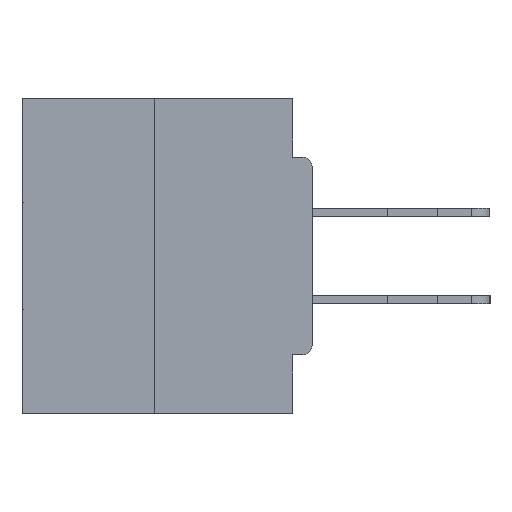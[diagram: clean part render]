
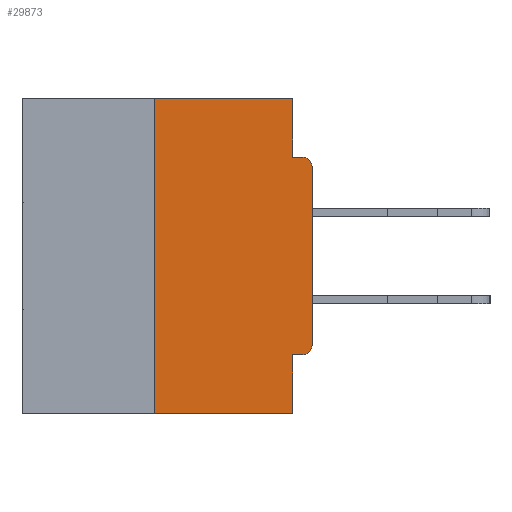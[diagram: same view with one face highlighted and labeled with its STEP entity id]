
A CAD part, left-side view. The second image highlights one B-rep face of the part: STEP entity #29873.
In plain terms, the highlighted planar face has unit normal (-1, 0, 0).
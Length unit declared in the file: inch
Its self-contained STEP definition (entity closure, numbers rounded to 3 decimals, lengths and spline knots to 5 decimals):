
#123 = DIRECTION ( 'NONE',  ( -1., 0., 0. ) ) ;
#266 = EDGE_CURVE ( 'NONE', #5417, #6742, #33635, .T. ) ;
#577 = PLANE ( 'NONE',  #16661 ) ;
#647 = VECTOR ( 'NONE', #34992, 39.37008 ) ;
#1261 = EDGE_CURVE ( 'NONE', #5051, #11264, #10518, .T. ) ;
#1477 = EDGE_CURVE ( 'NONE', #19738, #26381, #14347, .T. ) ;
#1625 = CARTESIAN_POINT ( 'NONE',  ( 0., 0., -0.0935 ) ) ;
#1950 = LINE ( 'NONE', #34639, #27022 ) ;
#1963 = ORIENTED_EDGE ( 'NONE', *, *, #266, .T. ) ;
#2167 = EDGE_LOOP ( 'NONE', ( #20236, #5785, #14823, #23198, #32314, #29704, #1963, #22966, #28393, #8883 ) ) ;
#2343 = CARTESIAN_POINT ( 'NONE',  ( 0., 0., -0.3915 ) ) ;
#3613 = EDGE_CURVE ( 'NONE', #35244, #5417, #31635, .T. ) ;
#3834 = VERTEX_POINT ( 'NONE', #25152 ) ;
#3877 = VERTEX_POINT ( 'NONE', #5016 ) ;
#4594 = CARTESIAN_POINT ( 'NONE',  ( 0., 0., 0. ) ) ;
#5016 = CARTESIAN_POINT ( 'NONE',  ( 0., 0.031, 0. ) ) ;
#5051 = VERTEX_POINT ( 'NONE', #23911 ) ;
#5258 = DIRECTION ( 'NONE',  ( 0., -1., 0. ) ) ;
#5417 = VERTEX_POINT ( 'NONE', #2343 ) ;
#5785 = ORIENTED_EDGE ( 'NONE', *, *, #28421, .F. ) ;
#5908 = DIRECTION ( 'NONE',  ( 0., 0., -1. ) ) ;
#6741 = VECTOR ( 'NONE', #5258, 39.37008 ) ;
#6742 = VERTEX_POINT ( 'NONE', #13669 ) ;
#6981 = VECTOR ( 'NONE', #13299, 39.37008 ) ;
#7478 = CARTESIAN_POINT ( 'NONE',  ( 0., 0.015, -0.4065 ) ) ;
#8329 = CARTESIAN_POINT ( 'NONE',  ( 0., 0.031, -0.5 ) ) ;
#8423 = CARTESIAN_POINT ( 'NONE',  ( 0., 0., -0.4065 ) ) ;
#8883 = ORIENTED_EDGE ( 'NONE', *, *, #29752, .F. ) ;
#10518 = LINE ( 'NONE', #1625, #6741 ) ;
#10946 = CARTESIAN_POINT ( 'NONE',  ( 0., 0.25, -0.5 ) ) ;
#11264 = VERTEX_POINT ( 'NONE', #30705 ) ;
#11385 = LINE ( 'NONE', #23202, #647 ) ;
#11564 = EDGE_CURVE ( 'NONE', #35244, #3834, #17111, .T. ) ;
#11834 = CARTESIAN_POINT ( 'NONE',  ( 0., 0.031, -0.5 ) ) ;
#12364 = DIRECTION ( 'NONE',  ( 0., 0., -1. ) ) ;
#13299 = DIRECTION ( 'NONE',  ( 0., 0., 1. ) ) ;
#13669 = CARTESIAN_POINT ( 'NONE',  ( 0., 0., -0.1085 ) ) ;
#14347 = LINE ( 'NONE', #35057, #15420 ) ;
#14405 = VECTOR ( 'NONE', #23130, 39.37008 ) ;
#14823 = ORIENTED_EDGE ( 'NONE', *, *, #1477, .T. ) ;
#15272 = CARTESIAN_POINT ( 'NONE',  ( 0., 0.46, 0. ) ) ;
#15420 = VECTOR ( 'NONE', #35260, 39.37008 ) ;
#15750 = VERTEX_POINT ( 'NONE', #18799 ) ;
#15954 = VECTOR ( 'NONE', #22295, 39.37008 ) ;
#16661 = AXIS2_PLACEMENT_3D ( 'NONE', #15272, #37117, #31308 ) ;
#17111 = LINE ( 'NONE', #8423, #14405 ) ;
#18195 = DIRECTION ( 'NONE',  ( -1., 0., 0. ) ) ;
#18752 = CARTESIAN_POINT ( 'NONE',  ( 0., 0.031, 0. ) ) ;
#18799 = CARTESIAN_POINT ( 'NONE',  ( 0., 0.25, 0. ) ) ;
#19552 = DIRECTION ( 'NONE',  ( 0., -1., 0. ) ) ;
#19738 = VERTEX_POINT ( 'NONE', #10946 ) ;
#20131 = LINE ( 'NONE', #8329, #15954 ) ;
#20236 = ORIENTED_EDGE ( 'NONE', *, *, #37230, .F. ) ;
#20635 = CARTESIAN_POINT ( 'NONE',  ( 0., 0.015, -0.1085 ) ) ;
#22032 = FACE_OUTER_BOUND ( 'NONE', #2167, .T. ) ;
#22295 = DIRECTION ( 'NONE',  ( 0., 0., -1. ) ) ;
#22966 = ORIENTED_EDGE ( 'NONE', *, *, #31296, .T. ) ;
#23130 = DIRECTION ( 'NONE',  ( 0., 1., 0. ) ) ;
#23198 = ORIENTED_EDGE ( 'NONE', *, *, #26671, .F. ) ;
#23202 = CARTESIAN_POINT ( 'NONE',  ( 0., 0.25, 0. ) ) ;
#23911 = CARTESIAN_POINT ( 'NONE',  ( 0., 0.031, -0.0935 ) ) ;
#25152 = CARTESIAN_POINT ( 'NONE',  ( 0., 0.031, -0.4065 ) ) ;
#26381 = VERTEX_POINT ( 'NONE', #11834 ) ;
#26671 = EDGE_CURVE ( 'NONE', #3834, #26381, #20131, .T. ) ;
#26912 = DIRECTION ( 'NONE',  ( 0., 0., -1. ) ) ;
#27022 = VECTOR ( 'NONE', #19552, 39.37008 ) ;
#28393 = ORIENTED_EDGE ( 'NONE', *, *, #1261, .F. ) ;
#28421 = EDGE_CURVE ( 'NONE', #19738, #15750, #11385, .T. ) ;
#29704 = ORIENTED_EDGE ( 'NONE', *, *, #3613, .T. ) ;
#29752 = EDGE_CURVE ( 'NONE', #3877, #5051, #33640, .T. ) ;
#29873 = ADVANCED_FACE ( 'NONE', ( #22032 ), #577, .F. ) ;
#30015 = CARTESIAN_POINT ( 'NONE',  ( 0., 0.015, -0.3915 ) ) ;
#30705 = CARTESIAN_POINT ( 'NONE',  ( 0., 0.015, -0.0935 ) ) ;
#31296 = EDGE_CURVE ( 'NONE', #6742, #11264, #32111, .T. ) ;
#31308 = DIRECTION ( 'NONE',  ( 0., 0., -1. ) ) ;
#31635 = CIRCLE ( 'NONE', #36589, 0.015 ) ;
#32111 = CIRCLE ( 'NONE', #33958, 0.015 ) ;
#32314 = ORIENTED_EDGE ( 'NONE', *, *, #11564, .F. ) ;
#33635 = LINE ( 'NONE', #4594, #6981 ) ;
#33640 = LINE ( 'NONE', #18752, #36467 ) ;
#33958 = AXIS2_PLACEMENT_3D ( 'NONE', #20635, #123, #5908 ) ;
#34639 = CARTESIAN_POINT ( 'NONE',  ( 0., 0.46, 0. ) ) ;
#34992 = DIRECTION ( 'NONE',  ( 0., 0., 1. ) ) ;
#35057 = CARTESIAN_POINT ( 'NONE',  ( 0., 0.46, -0.5 ) ) ;
#35244 = VERTEX_POINT ( 'NONE', #7478 ) ;
#35260 = DIRECTION ( 'NONE',  ( 0., -1., 0. ) ) ;
#36467 = VECTOR ( 'NONE', #12364, 39.37008 ) ;
#36589 = AXIS2_PLACEMENT_3D ( 'NONE', #30015, #18195, #26912 ) ;
#37117 = DIRECTION ( 'NONE',  ( 1., 0., 0. ) ) ;
#37230 = EDGE_CURVE ( 'NONE', #15750, #3877, #1950, .T. ) ;
